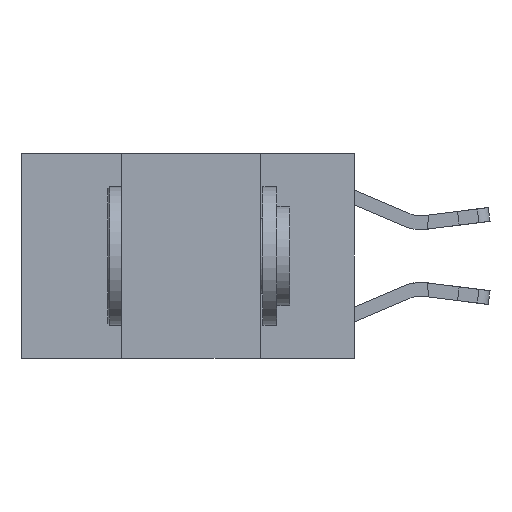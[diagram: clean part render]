
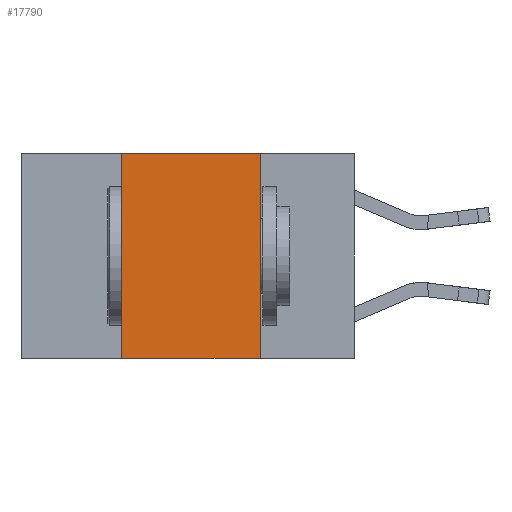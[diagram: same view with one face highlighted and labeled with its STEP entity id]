
A CAD part, left-side view. The second image highlights one B-rep face of the part: STEP entity #17790.
In plain terms, the highlighted planar face has unit normal (-1, 0, 0).
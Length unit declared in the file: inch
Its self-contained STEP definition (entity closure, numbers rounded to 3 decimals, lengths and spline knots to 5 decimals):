
#314 = CARTESIAN_POINT ( 'NONE',  ( 0., 0.6, -0.37 ) ) ;
#774 = EDGE_CURVE ( 'NONE', #1211, #13524, #20293, .T. ) ;
#1211 = VERTEX_POINT ( 'NONE', #7975 ) ;
#1789 = CARTESIAN_POINT ( 'NONE',  ( 0., 0.6, 0. ) ) ;
#2086 = VECTOR ( 'NONE', #3517, 39.37008 ) ;
#2615 = DIRECTION ( 'NONE',  ( 0., -1., 0. ) ) ;
#2855 = VECTOR ( 'NONE', #4868, 39.37008 ) ;
#3469 = EDGE_CURVE ( 'NONE', #1211, #12046, #19435, .T. ) ;
#3517 = DIRECTION ( 'NONE',  ( 0., -1., 0. ) ) ;
#4768 = DIRECTION ( 'NONE',  ( 0., 0., -1. ) ) ;
#4868 = DIRECTION ( 'NONE',  ( 0., 0., -1. ) ) ;
#6150 = VERTEX_POINT ( 'NONE', #21230 ) ;
#6518 = CARTESIAN_POINT ( 'NONE',  ( 0., 0.42, 0. ) ) ;
#6980 = ORIENTED_EDGE ( 'NONE', *, *, #22021, .F. ) ;
#7150 = VECTOR ( 'NONE', #2615, 39.37008 ) ;
#7322 = DIRECTION ( 'NONE',  ( 1., 0., 0. ) ) ;
#7975 = CARTESIAN_POINT ( 'NONE',  ( 0., 0.42, -0.37 ) ) ;
#8941 = ORIENTED_EDGE ( 'NONE', *, *, #774, .T. ) ;
#9249 = FACE_OUTER_BOUND ( 'NONE', #10528, .T. ) ;
#10528 = EDGE_LOOP ( 'NONE', ( #19897, #6980, #19711, #8941 ) ) ;
#10859 = VECTOR ( 'NONE', #15086, 39.37008 ) ;
#11389 = CARTESIAN_POINT ( 'NONE',  ( 0., 0.42, 0. ) ) ;
#12046 = VERTEX_POINT ( 'NONE', #6518 ) ;
#13176 = LINE ( 'NONE', #22811, #2855 ) ;
#13524 = VERTEX_POINT ( 'NONE', #17927 ) ;
#14757 = PLANE ( 'NONE',  #23710 ) ;
#15086 = DIRECTION ( 'NONE',  ( 0., 0., 1. ) ) ;
#17559 = LINE ( 'NONE', #1789, #2086 ) ;
#17790 = ADVANCED_FACE ( 'NONE', ( #9249 ), #14757, .F. ) ;
#17927 = CARTESIAN_POINT ( 'NONE',  ( 0., 0.17, -0.37 ) ) ;
#19435 = LINE ( 'NONE', #11389, #10859 ) ;
#19711 = ORIENTED_EDGE ( 'NONE', *, *, #3469, .F. ) ;
#19897 = ORIENTED_EDGE ( 'NONE', *, *, #20837, .F. ) ;
#20293 = LINE ( 'NONE', #314, #7150 ) ;
#20837 = EDGE_CURVE ( 'NONE', #6150, #13524, #13176, .T. ) ;
#21230 = CARTESIAN_POINT ( 'NONE',  ( 0., 0.17, 0. ) ) ;
#22021 = EDGE_CURVE ( 'NONE', #12046, #6150, #17559, .T. ) ;
#22811 = CARTESIAN_POINT ( 'NONE',  ( 0., 0.17, 0. ) ) ;
#23710 = AXIS2_PLACEMENT_3D ( 'NONE', #24889, #7322, #4768 ) ;
#24889 = CARTESIAN_POINT ( 'NONE',  ( 0., 0.6, 0. ) ) ;
